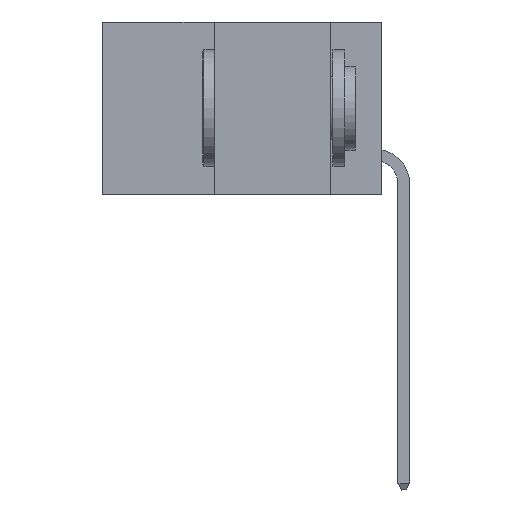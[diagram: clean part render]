
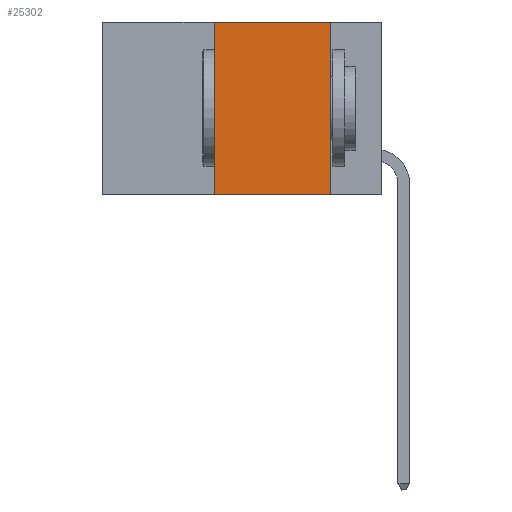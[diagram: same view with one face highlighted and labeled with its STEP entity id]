
A CAD part, left-side view. The second image highlights one B-rep face of the part: STEP entity #25302.
In plain terms, the highlighted planar face has unit normal (-1, 0, 0).
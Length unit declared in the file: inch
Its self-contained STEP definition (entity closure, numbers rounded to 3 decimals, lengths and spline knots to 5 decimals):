
#1331 = EDGE_CURVE ( 'NONE', #30988, #24233, #25835, .T. ) ;
#2203 = VECTOR ( 'NONE', #7945, 39.37008 ) ;
#4111 = DIRECTION ( 'NONE',  ( 0., 0., 1. ) ) ;
#4291 = CARTESIAN_POINT ( 'NONE',  ( 0., 0.6, 0. ) ) ;
#5831 = CARTESIAN_POINT ( 'NONE',  ( 0., 0.36, -0.37 ) ) ;
#6413 = CARTESIAN_POINT ( 'NONE',  ( 0., 0.11, 0. ) ) ;
#6718 = FACE_OUTER_BOUND ( 'NONE', #24937, .T. ) ;
#7795 = VECTOR ( 'NONE', #4111, 39.37008 ) ;
#7945 = DIRECTION ( 'NONE',  ( 0., -1., 0. ) ) ;
#9604 = CARTESIAN_POINT ( 'NONE',  ( 0., 0.6, -0.37 ) ) ;
#10854 = ORIENTED_EDGE ( 'NONE', *, *, #1331, .F. ) ;
#11055 = ORIENTED_EDGE ( 'NONE', *, *, #43459, .F. ) ;
#12172 = VECTOR ( 'NONE', #29910, 39.37008 ) ;
#12834 = DIRECTION ( 'NONE',  ( 0., -1., 0. ) ) ;
#12839 = PLANE ( 'NONE',  #25876 ) ;
#12985 = VERTEX_POINT ( 'NONE', #5831 ) ;
#13121 = DIRECTION ( 'NONE',  ( 0., 0., -1. ) ) ;
#13558 = LINE ( 'NONE', #20544, #7795 ) ;
#16360 = CARTESIAN_POINT ( 'NONE',  ( 0., 0.6, 0. ) ) ;
#20494 = EDGE_CURVE ( 'NONE', #12985, #24233, #29130, .T. ) ;
#20544 = CARTESIAN_POINT ( 'NONE',  ( 0., 0.36, 0. ) ) ;
#24216 = CARTESIAN_POINT ( 'NONE',  ( 0., 0.11, 0. ) ) ;
#24233 = VERTEX_POINT ( 'NONE', #38843 ) ;
#24937 = EDGE_LOOP ( 'NONE', ( #10854, #11055, #37305, #32317 ) ) ;
#25302 = ADVANCED_FACE ( 'NONE', ( #6718 ), #12839, .F. ) ;
#25835 = LINE ( 'NONE', #6413, #12172 ) ;
#25876 = AXIS2_PLACEMENT_3D ( 'NONE', #16360, #36313, #13121 ) ;
#27354 = CARTESIAN_POINT ( 'NONE',  ( 0., 0.36, 0. ) ) ;
#29130 = LINE ( 'NONE', #9604, #33314 ) ;
#29910 = DIRECTION ( 'NONE',  ( 0., 0., -1. ) ) ;
#30988 = VERTEX_POINT ( 'NONE', #24216 ) ;
#32169 = LINE ( 'NONE', #4291, #2203 ) ;
#32317 = ORIENTED_EDGE ( 'NONE', *, *, #20494, .T. ) ;
#33314 = VECTOR ( 'NONE', #12834, 39.37008 ) ;
#35228 = EDGE_CURVE ( 'NONE', #12985, #43379, #13558, .T. ) ;
#36313 = DIRECTION ( 'NONE',  ( 1., 0., 0. ) ) ;
#37305 = ORIENTED_EDGE ( 'NONE', *, *, #35228, .F. ) ;
#38843 = CARTESIAN_POINT ( 'NONE',  ( 0., 0.11, -0.37 ) ) ;
#43379 = VERTEX_POINT ( 'NONE', #27354 ) ;
#43459 = EDGE_CURVE ( 'NONE', #43379, #30988, #32169, .T. ) ;
